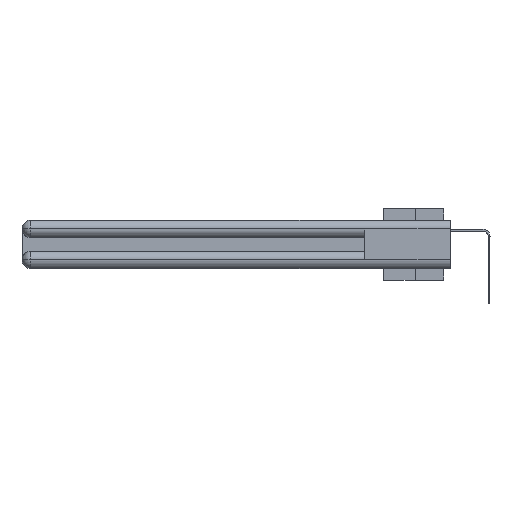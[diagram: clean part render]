
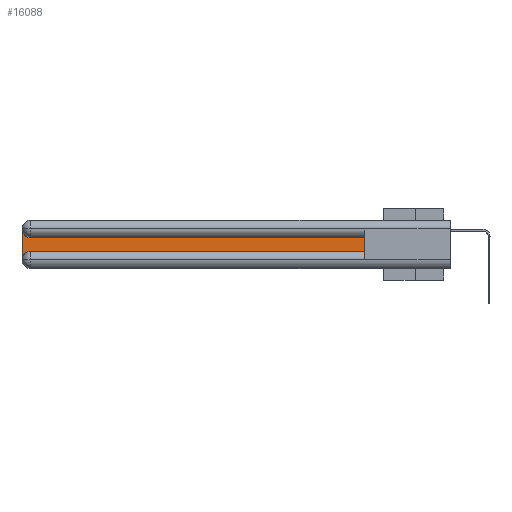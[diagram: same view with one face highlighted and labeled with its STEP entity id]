
A CAD part, left-side view. The second image highlights one B-rep face of the part: STEP entity #16088.
In plain terms, the highlighted planar face has unit normal (-1, 0, 0).
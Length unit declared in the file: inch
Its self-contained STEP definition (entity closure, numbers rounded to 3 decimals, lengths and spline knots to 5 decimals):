
#449 = ORIENTED_EDGE ( 'NONE', *, *, #31381, .T. ) ;
#613 = DIRECTION ( 'NONE',  ( 1., 0., 0. ) ) ;
#1923 = DIRECTION ( 'NONE',  ( 0., 0., 1. ) ) ;
#3048 = VECTOR ( 'NONE', #1923, 39.37008 ) ;
#3553 = AXIS2_PLACEMENT_3D ( 'NONE', #10963, #25324, #11087 ) ;
#4974 = DIRECTION ( 'NONE',  ( 0., 0., -1. ) ) ;
#5159 = VERTEX_POINT ( 'NONE', #27218 ) ;
#9229 = ORIENTED_EDGE ( 'NONE', *, *, #30308, .T. ) ;
#9372 = ORIENTED_EDGE ( 'NONE', *, *, #21530, .T. ) ;
#9592 = LINE ( 'NONE', #23207, #31714 ) ;
#9740 = VERTEX_POINT ( 'NONE', #30315 ) ;
#10541 = LINE ( 'NONE', #21395, #3048 ) ;
#10963 = CARTESIAN_POINT ( 'NONE',  ( 0.075, 2.94, -0.0625 ) ) ;
#11087 = DIRECTION ( 'NONE',  ( 0., 0., -1. ) ) ;
#11370 = DIRECTION ( 'NONE',  ( 0., 1., 0. ) ) ;
#11447 = CARTESIAN_POINT ( 'NONE',  ( 0.075, 2.94, -0.2175 ) ) ;
#11922 = AXIS2_PLACEMENT_3D ( 'NONE', #14400, #613, #14276 ) ;
#13484 = VERTEX_POINT ( 'NONE', #28515 ) ;
#14201 = CARTESIAN_POINT ( 'NONE',  ( 0.075, 0.6, -0.1225 ) ) ;
#14276 = DIRECTION ( 'NONE',  ( 0., 0., -1. ) ) ;
#14400 = CARTESIAN_POINT ( 'NONE',  ( 0.075, 2.94, -0.2775 ) ) ;
#16088 = ADVANCED_FACE ( 'NONE', ( #34890 ), #33236, .F. ) ;
#17510 = DIRECTION ( 'NONE',  ( 0., 0., -1. ) ) ;
#18666 = DIRECTION ( 'NONE',  ( 0., -1., 0. ) ) ;
#18711 = VERTEX_POINT ( 'NONE', #11447 ) ;
#18940 = LINE ( 'NONE', #35591, #21626 ) ;
#20652 = LINE ( 'NONE', #14201, #29508 ) ;
#21395 = CARTESIAN_POINT ( 'NONE',  ( 0.075, 0.6, -0.2175 ) ) ;
#21530 = EDGE_CURVE ( 'NONE', #18711, #9740, #18940, .T. ) ;
#21626 = VECTOR ( 'NONE', #18666, 39.37008 ) ;
#22348 = CARTESIAN_POINT ( 'NONE',  ( 0.075, 3., -0.1225 ) ) ;
#22585 = EDGE_CURVE ( 'NONE', #31773, #5159, #20652, .T. ) ;
#23023 = CIRCLE ( 'NONE', #11922, 0.06 ) ;
#23207 = CARTESIAN_POINT ( 'NONE',  ( 0.075, 3., -0.2175 ) ) ;
#23577 = ORIENTED_EDGE ( 'NONE', *, *, #25989, .T. ) ;
#23871 = CARTESIAN_POINT ( 'NONE',  ( 0.075, 3., -0.0625 ) ) ;
#24502 = CIRCLE ( 'NONE', #3553, 0.06 ) ;
#24595 = EDGE_LOOP ( 'NONE', ( #29870, #23577, #9229, #32584, #9372, #449 ) ) ;
#25324 = DIRECTION ( 'NONE',  ( 1., 0., 0. ) ) ;
#25989 = EDGE_CURVE ( 'NONE', #5159, #32973, #24502, .T. ) ;
#27218 = CARTESIAN_POINT ( 'NONE',  ( 0.075, 2.94, -0.1225 ) ) ;
#27701 = DIRECTION ( 'NONE',  ( 1., 0., 0. ) ) ;
#28515 = CARTESIAN_POINT ( 'NONE',  ( 0.075, 3., -0.2775 ) ) ;
#29298 = CARTESIAN_POINT ( 'NONE',  ( 0.075, 0.6, -0.1225 ) ) ;
#29508 = VECTOR ( 'NONE', #11370, 39.37008 ) ;
#29870 = ORIENTED_EDGE ( 'NONE', *, *, #22585, .T. ) ;
#30308 = EDGE_CURVE ( 'NONE', #32973, #13484, #9592, .T. ) ;
#30315 = CARTESIAN_POINT ( 'NONE',  ( 0.075, 0.6, -0.2175 ) ) ;
#31381 = EDGE_CURVE ( 'NONE', #9740, #31773, #10541, .T. ) ;
#31714 = VECTOR ( 'NONE', #17510, 39.37008 ) ;
#31773 = VERTEX_POINT ( 'NONE', #29298 ) ;
#31942 = AXIS2_PLACEMENT_3D ( 'NONE', #22348, #27701, #4974 ) ;
#32584 = ORIENTED_EDGE ( 'NONE', *, *, #36289, .T. ) ;
#32973 = VERTEX_POINT ( 'NONE', #23871 ) ;
#33236 = PLANE ( 'NONE',  #31942 ) ;
#34890 = FACE_OUTER_BOUND ( 'NONE', #24595, .T. ) ;
#35591 = CARTESIAN_POINT ( 'NONE',  ( 0.075, 0.6, -0.2175 ) ) ;
#36289 = EDGE_CURVE ( 'NONE', #13484, #18711, #23023, .T. ) ;
